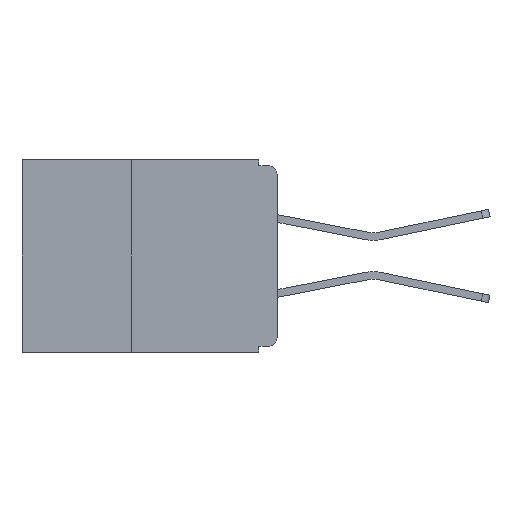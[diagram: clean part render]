
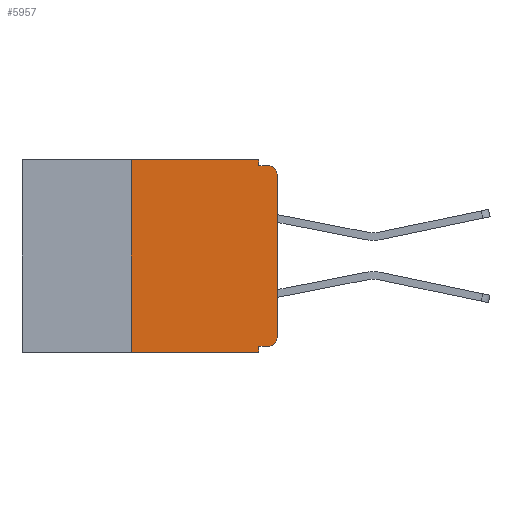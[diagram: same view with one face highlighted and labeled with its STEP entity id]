
A CAD part, left-side view. The second image highlights one B-rep face of the part: STEP entity #5957.
In plain terms, the highlighted planar face has unit normal (-1, 0, 0).
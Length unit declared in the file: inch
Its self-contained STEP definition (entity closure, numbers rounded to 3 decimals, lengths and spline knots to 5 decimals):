
#637 = LINE ( 'NONE', #14169, #28911 ) ;
#1638 = CARTESIAN_POINT ( 'NONE',  ( 0., 0.015, -0.305 ) ) ;
#1904 = ORIENTED_EDGE ( 'NONE', *, *, #32388, .F. ) ;
#1947 = VERTEX_POINT ( 'NONE', #12106 ) ;
#3346 = EDGE_CURVE ( 'NONE', #22314, #18439, #21665, .T. ) ;
#4094 = LINE ( 'NONE', #16055, #32033 ) ;
#4344 = VERTEX_POINT ( 'NONE', #27655 ) ;
#4539 = DIRECTION ( 'NONE',  ( 0., 0., -1. ) ) ;
#4919 = VERTEX_POINT ( 'NONE', #23409 ) ;
#5046 = EDGE_CURVE ( 'NONE', #33085, #7041, #27851, .T. ) ;
#5526 = ORIENTED_EDGE ( 'NONE', *, *, #6918, .T. ) ;
#5957 = ADVANCED_FACE ( 'NONE', ( #23238 ), #6311, .F. ) ;
#6311 = PLANE ( 'NONE',  #9144 ) ;
#6734 = VECTOR ( 'NONE', #9545, 39.37008 ) ;
#6906 = LINE ( 'NONE', #11316, #20561 ) ;
#6918 = EDGE_CURVE ( 'NONE', #20390, #7041, #26922, .T. ) ;
#7041 = VERTEX_POINT ( 'NONE', #10949 ) ;
#7701 = ORIENTED_EDGE ( 'NONE', *, *, #10883, .T. ) ;
#7872 = VERTEX_POINT ( 'NONE', #17564 ) ;
#9113 = DIRECTION ( 'NONE',  ( 0., 0., -1. ) ) ;
#9123 = LINE ( 'NONE', #26958, #22709 ) ;
#9144 = AXIS2_PLACEMENT_3D ( 'NONE', #11717, #25328, #9113 ) ;
#9237 = AXIS2_PLACEMENT_3D ( 'NONE', #16681, #35222, #19402 ) ;
#9545 = DIRECTION ( 'NONE',  ( 0., 0., 1. ) ) ;
#10195 = EDGE_CURVE ( 'NONE', #18439, #4344, #6906, .T. ) ;
#10271 = ORIENTED_EDGE ( 'NONE', *, *, #23012, .F. ) ;
#10489 = CARTESIAN_POINT ( 'NONE',  ( 0., 0., -0.305 ) ) ;
#10731 = ORIENTED_EDGE ( 'NONE', *, *, #3346, .T. ) ;
#10883 = EDGE_CURVE ( 'NONE', #4344, #4919, #12834, .T. ) ;
#10949 = CARTESIAN_POINT ( 'NONE',  ( 0., 0.031, -0.33 ) ) ;
#11316 = CARTESIAN_POINT ( 'NONE',  ( 0., 0., 0. ) ) ;
#11717 = CARTESIAN_POINT ( 'NONE',  ( 0., 0.437, 0. ) ) ;
#12106 = CARTESIAN_POINT ( 'NONE',  ( 0., 0.031, 0. ) ) ;
#12416 = EDGE_CURVE ( 'NONE', #20390, #7872, #25969, .T. ) ;
#12532 = VECTOR ( 'NONE', #31808, 39.37008 ) ;
#12834 = CIRCLE ( 'NONE', #9237, 0.015 ) ;
#13065 = DIRECTION ( 'NONE',  ( 0., 0., -1. ) ) ;
#13379 = DIRECTION ( 'NONE',  ( 0., -1., 0. ) ) ;
#14077 = ORIENTED_EDGE ( 'NONE', *, *, #10195, .T. ) ;
#14169 = CARTESIAN_POINT ( 'NONE',  ( 0., 0., -0.32 ) ) ;
#14260 = EDGE_CURVE ( 'NONE', #1947, #34398, #20476, .T. ) ;
#16055 = CARTESIAN_POINT ( 'NONE',  ( 0., 0.437, 0. ) ) ;
#16668 = ORIENTED_EDGE ( 'NONE', *, *, #14260, .F. ) ;
#16681 = CARTESIAN_POINT ( 'NONE',  ( 0., 0.015, -0.025 ) ) ;
#16929 = DIRECTION ( 'NONE',  ( 0., 1., 0. ) ) ;
#17084 = AXIS2_PLACEMENT_3D ( 'NONE', #1638, #20956, #4539 ) ;
#17564 = CARTESIAN_POINT ( 'NONE',  ( 0., 0.25, 0. ) ) ;
#17631 = CARTESIAN_POINT ( 'NONE',  ( 0., 0.031, 0. ) ) ;
#17741 = DIRECTION ( 'NONE',  ( 0., 0., -1. ) ) ;
#18200 = EDGE_CURVE ( 'NONE', #22314, #33085, #637, .T. ) ;
#18439 = VERTEX_POINT ( 'NONE', #10489 ) ;
#19402 = DIRECTION ( 'NONE',  ( 0., 0., -1. ) ) ;
#20052 = ORIENTED_EDGE ( 'NONE', *, *, #5046, .F. ) ;
#20390 = VERTEX_POINT ( 'NONE', #28616 ) ;
#20476 = LINE ( 'NONE', #17631, #28394 ) ;
#20561 = VECTOR ( 'NONE', #30231, 39.37008 ) ;
#20774 = VECTOR ( 'NONE', #13065, 39.37008 ) ;
#20956 = DIRECTION ( 'NONE',  ( -1., 0., 0. ) ) ;
#21665 = CIRCLE ( 'NONE', #17084, 0.015 ) ;
#21766 = CARTESIAN_POINT ( 'NONE',  ( 0., 0.031, -0.32 ) ) ;
#22314 = VERTEX_POINT ( 'NONE', #31939 ) ;
#22709 = VECTOR ( 'NONE', #13379, 39.37008 ) ;
#23012 = EDGE_CURVE ( 'NONE', #7872, #1947, #4094, .T. ) ;
#23238 = FACE_OUTER_BOUND ( 'NONE', #32387, .T. ) ;
#23409 = CARTESIAN_POINT ( 'NONE',  ( 0., 0.015, -0.01 ) ) ;
#23880 = CARTESIAN_POINT ( 'NONE',  ( 0., 0.031, -0.33 ) ) ;
#24215 = DIRECTION ( 'NONE',  ( 0., -1., 0. ) ) ;
#25328 = DIRECTION ( 'NONE',  ( 1., 0., 0. ) ) ;
#25969 = LINE ( 'NONE', #33773, #6734 ) ;
#26922 = LINE ( 'NONE', #34425, #12532 ) ;
#26958 = CARTESIAN_POINT ( 'NONE',  ( 0., 0., -0.01 ) ) ;
#27655 = CARTESIAN_POINT ( 'NONE',  ( 0., 0., -0.025 ) ) ;
#27851 = LINE ( 'NONE', #23880, #20774 ) ;
#28394 = VECTOR ( 'NONE', #17741, 39.37008 ) ;
#28616 = CARTESIAN_POINT ( 'NONE',  ( 0., 0.25, -0.33 ) ) ;
#28911 = VECTOR ( 'NONE', #16929, 39.37008 ) ;
#29633 = CARTESIAN_POINT ( 'NONE',  ( 0., 0.031, -0.01 ) ) ;
#30231 = DIRECTION ( 'NONE',  ( 0., 0., 1. ) ) ;
#30455 = ORIENTED_EDGE ( 'NONE', *, *, #18200, .F. ) ;
#31808 = DIRECTION ( 'NONE',  ( 0., -1., 0. ) ) ;
#31939 = CARTESIAN_POINT ( 'NONE',  ( 0., 0.015, -0.32 ) ) ;
#32033 = VECTOR ( 'NONE', #24215, 39.37008 ) ;
#32387 = EDGE_LOOP ( 'NONE', ( #14077, #7701, #1904, #16668, #10271, #32452, #5526, #20052, #30455, #10731 ) ) ;
#32388 = EDGE_CURVE ( 'NONE', #34398, #4919, #9123, .T. ) ;
#32452 = ORIENTED_EDGE ( 'NONE', *, *, #12416, .F. ) ;
#33085 = VERTEX_POINT ( 'NONE', #21766 ) ;
#33773 = CARTESIAN_POINT ( 'NONE',  ( 0., 0.25, -0.33 ) ) ;
#34398 = VERTEX_POINT ( 'NONE', #29633 ) ;
#34425 = CARTESIAN_POINT ( 'NONE',  ( 0., 0.437, -0.33 ) ) ;
#35222 = DIRECTION ( 'NONE',  ( -1., 0., 0. ) ) ;
